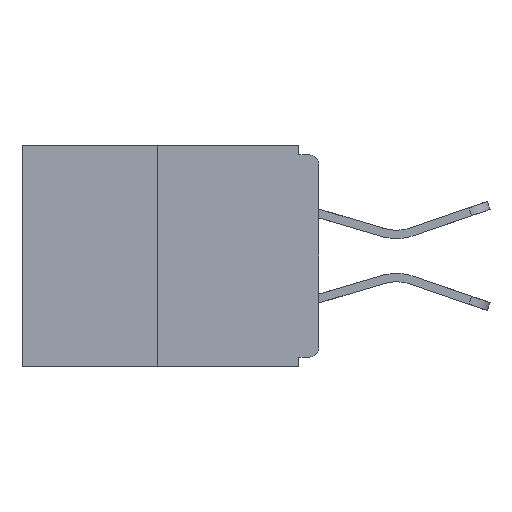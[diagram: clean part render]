
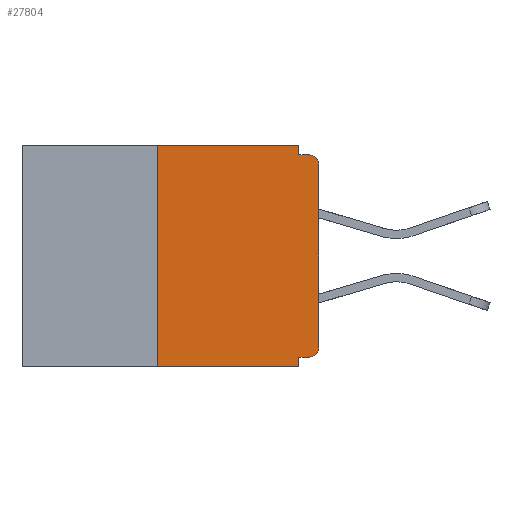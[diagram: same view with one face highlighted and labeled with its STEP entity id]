
A CAD part, left-side view. The second image highlights one B-rep face of the part: STEP entity #27804.
In plain terms, the highlighted planar face has unit normal (-1, 0, 0).
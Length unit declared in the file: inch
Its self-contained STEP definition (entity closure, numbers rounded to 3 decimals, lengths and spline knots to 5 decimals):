
#39 = CIRCLE ( 'NONE', #18416, 0.015 ) ;
#149 = DIRECTION ( 'NONE',  ( 0., -1., 0. ) ) ;
#281 = EDGE_CURVE ( 'NONE', #23580, #8240, #21031, .T. ) ;
#304 = LINE ( 'NONE', #22460, #16641 ) ;
#689 = EDGE_CURVE ( 'NONE', #23580, #14643, #39, .T. ) ;
#810 = CARTESIAN_POINT ( 'NONE',  ( 0., 0.015, -0.313 ) ) ;
#905 = LINE ( 'NONE', #10341, #25200 ) ;
#1514 = VECTOR ( 'NONE', #18397, 39.37008 ) ;
#1520 = VECTOR ( 'NONE', #2218, 39.37008 ) ;
#1565 = ORIENTED_EDGE ( 'NONE', *, *, #689, .T. ) ;
#1851 = CARTESIAN_POINT ( 'NONE',  ( 0., 0.031, -0.343 ) ) ;
#2218 = DIRECTION ( 'NONE',  ( 0., 1., 0. ) ) ;
#3046 = VERTEX_POINT ( 'NONE', #20860 ) ;
#3131 = ORIENTED_EDGE ( 'NONE', *, *, #281, .F. ) ;
#3757 = EDGE_CURVE ( 'NONE', #13408, #27466, #7665, .T. ) ;
#4897 = VECTOR ( 'NONE', #25227, 39.37008 ) ;
#5149 = ORIENTED_EDGE ( 'NONE', *, *, #27242, .T. ) ;
#5694 = DIRECTION ( 'NONE',  ( -1., 0., 0. ) ) ;
#6378 = ORIENTED_EDGE ( 'NONE', *, *, #14802, .T. ) ;
#6762 = CARTESIAN_POINT ( 'NONE',  ( 0., 0., -0.313 ) ) ;
#6844 = CARTESIAN_POINT ( 'NONE',  ( 0., 0.031, 0. ) ) ;
#7200 = VECTOR ( 'NONE', #15541, 39.37008 ) ;
#7251 = CARTESIAN_POINT ( 'NONE',  ( 0., 0.46, 0. ) ) ;
#7665 = LINE ( 'NONE', #6844, #1514 ) ;
#7896 = EDGE_CURVE ( 'NONE', #23312, #13408, #905, .T. ) ;
#8240 = VERTEX_POINT ( 'NONE', #18395 ) ;
#8616 = DIRECTION ( 'NONE',  ( 0., 0., 1. ) ) ;
#8944 = CARTESIAN_POINT ( 'NONE',  ( 0., 0.031, -0.343 ) ) ;
#9494 = DIRECTION ( 'NONE',  ( -1., 0., 0. ) ) ;
#9908 = VECTOR ( 'NONE', #149, 39.37008 ) ;
#10241 = DIRECTION ( 'NONE',  ( 0., -1., 0. ) ) ;
#10341 = CARTESIAN_POINT ( 'NONE',  ( 0., 0.46, 0. ) ) ;
#10363 = ORIENTED_EDGE ( 'NONE', *, *, #3757, .F. ) ;
#10874 = CARTESIAN_POINT ( 'NONE',  ( 0., 0., 0. ) ) ;
#11802 = DIRECTION ( 'NONE',  ( 0., -1., 0. ) ) ;
#11835 = DIRECTION ( 'NONE',  ( 0., 0., -1. ) ) ;
#11926 = VECTOR ( 'NONE', #11802, 39.37008 ) ;
#11958 = DIRECTION ( 'NONE',  ( 1., 0., 0. ) ) ;
#12122 = CARTESIAN_POINT ( 'NONE',  ( 0., 0.015, -0.03 ) ) ;
#12354 = PLANE ( 'NONE',  #18816 ) ;
#12966 = ORIENTED_EDGE ( 'NONE', *, *, #27205, .F. ) ;
#13022 = VERTEX_POINT ( 'NONE', #22155 ) ;
#13252 = EDGE_CURVE ( 'NONE', #8240, #17505, #28785, .T. ) ;
#13280 = CARTESIAN_POINT ( 'NONE',  ( 0., 0.031, -0.015 ) ) ;
#13408 = VERTEX_POINT ( 'NONE', #18653 ) ;
#14063 = EDGE_CURVE ( 'NONE', #3046, #29293, #19323, .T. ) ;
#14195 = CARTESIAN_POINT ( 'NONE',  ( 0., 0.015, -0.328 ) ) ;
#14643 = VERTEX_POINT ( 'NONE', #6762 ) ;
#14802 = EDGE_CURVE ( 'NONE', #13022, #17505, #15380, .T. ) ;
#15380 = LINE ( 'NONE', #16589, #9908 ) ;
#15511 = ORIENTED_EDGE ( 'NONE', *, *, #16463, .F. ) ;
#15541 = DIRECTION ( 'NONE',  ( 0., 0., 1. ) ) ;
#16110 = CARTESIAN_POINT ( 'NONE',  ( 0., 0., -0.328 ) ) ;
#16463 = EDGE_CURVE ( 'NONE', #27466, #29293, #28491, .T. ) ;
#16589 = CARTESIAN_POINT ( 'NONE',  ( 0., 0.46, -0.343 ) ) ;
#16641 = VECTOR ( 'NONE', #8616, 39.37008 ) ;
#17505 = VERTEX_POINT ( 'NONE', #8944 ) ;
#17995 = ORIENTED_EDGE ( 'NONE', *, *, #7896, .F. ) ;
#18395 = CARTESIAN_POINT ( 'NONE',  ( 0., 0.031, -0.328 ) ) ;
#18397 = DIRECTION ( 'NONE',  ( 0., 0., -1. ) ) ;
#18416 = AXIS2_PLACEMENT_3D ( 'NONE', #810, #5694, #21857 ) ;
#18653 = CARTESIAN_POINT ( 'NONE',  ( 0., 0.031, 0. ) ) ;
#18816 = AXIS2_PLACEMENT_3D ( 'NONE', #7251, #11958, #28468 ) ;
#19323 = CIRCLE ( 'NONE', #26977, 0.015 ) ;
#20860 = CARTESIAN_POINT ( 'NONE',  ( 0., 0., -0.03 ) ) ;
#21031 = LINE ( 'NONE', #16110, #1520 ) ;
#21857 = DIRECTION ( 'NONE',  ( 0., 0., -1. ) ) ;
#22155 = CARTESIAN_POINT ( 'NONE',  ( 0., 0.25, -0.343 ) ) ;
#22460 = CARTESIAN_POINT ( 'NONE',  ( 0., 0.25, 0. ) ) ;
#22792 = ORIENTED_EDGE ( 'NONE', *, *, #13252, .F. ) ;
#23312 = VERTEX_POINT ( 'NONE', #29424 ) ;
#23580 = VERTEX_POINT ( 'NONE', #14195 ) ;
#24719 = FACE_OUTER_BOUND ( 'NONE', #29091, .T. ) ;
#24742 = ORIENTED_EDGE ( 'NONE', *, *, #14063, .T. ) ;
#25068 = CARTESIAN_POINT ( 'NONE',  ( 0., 0.015, -0.015 ) ) ;
#25200 = VECTOR ( 'NONE', #10241, 39.37008 ) ;
#25227 = DIRECTION ( 'NONE',  ( 0., 0., -1. ) ) ;
#25428 = CARTESIAN_POINT ( 'NONE',  ( 0., 0., -0.015 ) ) ;
#26977 = AXIS2_PLACEMENT_3D ( 'NONE', #12122, #9494, #11835 ) ;
#27205 = EDGE_CURVE ( 'NONE', #13022, #23312, #304, .T. ) ;
#27242 = EDGE_CURVE ( 'NONE', #14643, #3046, #29639, .T. ) ;
#27466 = VERTEX_POINT ( 'NONE', #13280 ) ;
#27804 = ADVANCED_FACE ( 'NONE', ( #24719 ), #12354, .F. ) ;
#28468 = DIRECTION ( 'NONE',  ( 0., 0., -1. ) ) ;
#28491 = LINE ( 'NONE', #25428, #11926 ) ;
#28785 = LINE ( 'NONE', #1851, #4897 ) ;
#29091 = EDGE_LOOP ( 'NONE', ( #17995, #12966, #6378, #22792, #3131, #1565, #5149, #24742, #15511, #10363 ) ) ;
#29293 = VERTEX_POINT ( 'NONE', #25068 ) ;
#29424 = CARTESIAN_POINT ( 'NONE',  ( 0., 0.25, 0. ) ) ;
#29639 = LINE ( 'NONE', #10874, #7200 ) ;
